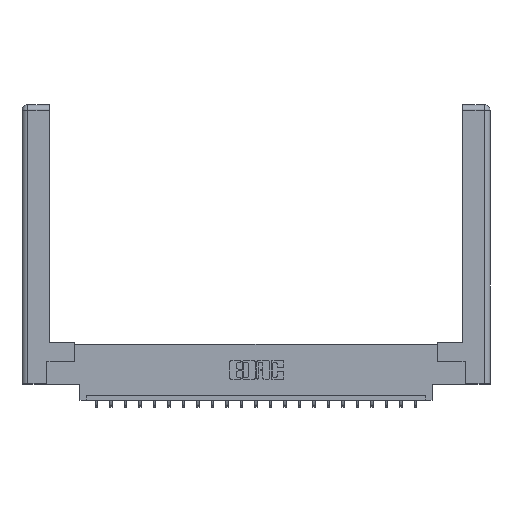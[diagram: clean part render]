
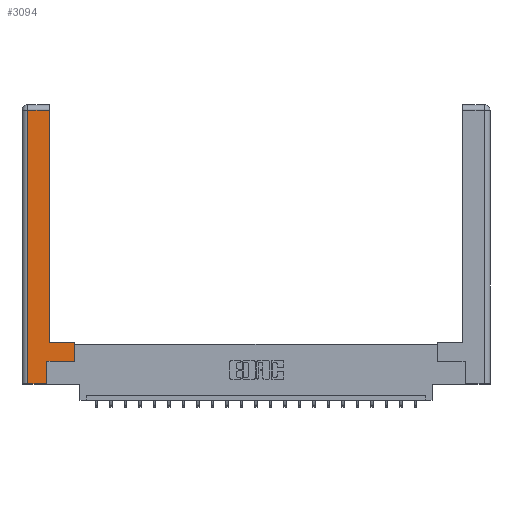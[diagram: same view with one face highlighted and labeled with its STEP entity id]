
A CAD part, top view. The second image highlights one B-rep face of the part: STEP entity #3094.
In plain terms, the highlighted planar face has unit normal (0, 0, 1).
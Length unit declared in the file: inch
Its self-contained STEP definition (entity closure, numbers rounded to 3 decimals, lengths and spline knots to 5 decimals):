
#520 = ORIENTED_EDGE ( 'NONE', *, *, #21738, .T. ) ;
#1027 = VECTOR ( 'NONE', #7647, 39.37008 ) ;
#1071 = CARTESIAN_POINT ( 'NONE',  ( 0.0615, 0., 0. ) ) ;
#1283 = VERTEX_POINT ( 'NONE', #9251 ) ;
#2079 = DIRECTION ( 'NONE',  ( -1., 0., 0. ) ) ;
#2188 = CARTESIAN_POINT ( 'NONE',  ( 0.265, 0., 0. ) ) ;
#2311 = LINE ( 'NONE', #14570, #1027 ) ;
#2562 = VERTEX_POINT ( 'NONE', #6169 ) ;
#2931 = CARTESIAN_POINT ( 'NONE',  ( 0.565, 0.245, 0. ) ) ;
#3043 = LINE ( 'NONE', #2931, #8749 ) ;
#3094 = ADVANCED_FACE ( 'NONE', ( #21939 ), #18521, .F. ) ;
#3102 = ORIENTED_EDGE ( 'NONE', *, *, #4562, .T. ) ;
#3155 = ORIENTED_EDGE ( 'NONE', *, *, #18211, .T. ) ;
#3216 = CARTESIAN_POINT ( 'NONE',  ( 0.0615, 0., 0. ) ) ;
#3499 = CARTESIAN_POINT ( 'NONE',  ( 0., 0., 0. ) ) ;
#3618 = CARTESIAN_POINT ( 'NONE',  ( 0.265, 0.245, 0. ) ) ;
#3730 = CARTESIAN_POINT ( 'NONE',  ( 0.565, 0.45, 0. ) ) ;
#3848 = LINE ( 'NONE', #20518, #10117 ) ;
#4331 = EDGE_CURVE ( 'NONE', #20703, #15228, #3043, .T. ) ;
#4562 = EDGE_CURVE ( 'NONE', #12860, #22203, #3848, .T. ) ;
#4608 = DIRECTION ( 'NONE',  ( 1., 0., 0. ) ) ;
#4748 = VECTOR ( 'NONE', #16927, 39.37008 ) ;
#5229 = LINE ( 'NONE', #17692, #18515 ) ;
#6169 = CARTESIAN_POINT ( 'NONE',  ( 0.265, 0., 0. ) ) ;
#7647 = DIRECTION ( 'NONE',  ( 0., 1., 0. ) ) ;
#8578 = EDGE_CURVE ( 'NONE', #22203, #13158, #17777, .T. ) ;
#8749 = VECTOR ( 'NONE', #4608, 39.37008 ) ;
#8993 = DIRECTION ( 'NONE',  ( 1., 0., 0. ) ) ;
#9251 = CARTESIAN_POINT ( 'NONE',  ( 0.295, 0.45, 0. ) ) ;
#9367 = ORIENTED_EDGE ( 'NONE', *, *, #14093, .T. ) ;
#10024 = CARTESIAN_POINT ( 'NONE',  ( 0.295, 2.94, 0. ) ) ;
#10117 = VECTOR ( 'NONE', #22296, 39.37008 ) ;
#10904 = CARTESIAN_POINT ( 'NONE',  ( 0.565, 0.245, 0. ) ) ;
#11083 = AXIS2_PLACEMENT_3D ( 'NONE', #3499, #19130, #13978 ) ;
#11696 = VERTEX_POINT ( 'NONE', #19020 ) ;
#12073 = LINE ( 'NONE', #2188, #21819 ) ;
#12860 = VERTEX_POINT ( 'NONE', #10024 ) ;
#13158 = VERTEX_POINT ( 'NONE', #3216 ) ;
#13437 = CARTESIAN_POINT ( 'NONE',  ( 0.295, 3., 0. ) ) ;
#13651 = ORIENTED_EDGE ( 'NONE', *, *, #18115, .T. ) ;
#13867 = ORIENTED_EDGE ( 'NONE', *, *, #19922, .T. ) ;
#13978 = DIRECTION ( 'NONE',  ( -1., 0., 0. ) ) ;
#14093 = EDGE_CURVE ( 'NONE', #15228, #11696, #17491, .T. ) ;
#14229 = LINE ( 'NONE', #13437, #4748 ) ;
#14570 = CARTESIAN_POINT ( 'NONE',  ( 0.265, 0.245, 0. ) ) ;
#15228 = VERTEX_POINT ( 'NONE', #10904 ) ;
#16819 = EDGE_LOOP ( 'NONE', ( #3155, #3102, #20586, #13651, #520, #18239, #9367, #13867 ) ) ;
#16927 = DIRECTION ( 'NONE',  ( 0., 1., 0. ) ) ;
#17176 = CARTESIAN_POINT ( 'NONE',  ( 0.0615, 2.94, 0. ) ) ;
#17216 = VECTOR ( 'NONE', #21932, 39.37008 ) ;
#17491 = LINE ( 'NONE', #3730, #20756 ) ;
#17676 = DIRECTION ( 'NONE',  ( 0., 1., 0. ) ) ;
#17692 = CARTESIAN_POINT ( 'NONE',  ( 0.295, 0.45, 0. ) ) ;
#17777 = LINE ( 'NONE', #1071, #17216 ) ;
#18115 = EDGE_CURVE ( 'NONE', #13158, #2562, #12073, .T. ) ;
#18211 = EDGE_CURVE ( 'NONE', #1283, #12860, #14229, .T. ) ;
#18239 = ORIENTED_EDGE ( 'NONE', *, *, #4331, .T. ) ;
#18515 = VECTOR ( 'NONE', #2079, 39.37008 ) ;
#18521 = PLANE ( 'NONE',  #11083 ) ;
#19020 = CARTESIAN_POINT ( 'NONE',  ( 0.565, 0.45, 0. ) ) ;
#19130 = DIRECTION ( 'NONE',  ( 0., 0., -1. ) ) ;
#19922 = EDGE_CURVE ( 'NONE', #11696, #1283, #5229, .T. ) ;
#20518 = CARTESIAN_POINT ( 'NONE',  ( 0.0615, 2.94, 0. ) ) ;
#20586 = ORIENTED_EDGE ( 'NONE', *, *, #8578, .T. ) ;
#20703 = VERTEX_POINT ( 'NONE', #3618 ) ;
#20756 = VECTOR ( 'NONE', #17676, 39.37008 ) ;
#21738 = EDGE_CURVE ( 'NONE', #2562, #20703, #2311, .T. ) ;
#21819 = VECTOR ( 'NONE', #8993, 39.37008 ) ;
#21932 = DIRECTION ( 'NONE',  ( 0., -1., 0. ) ) ;
#21939 = FACE_OUTER_BOUND ( 'NONE', #16819, .T. ) ;
#22203 = VERTEX_POINT ( 'NONE', #17176 ) ;
#22296 = DIRECTION ( 'NONE',  ( -1., 0., 0. ) ) ;
